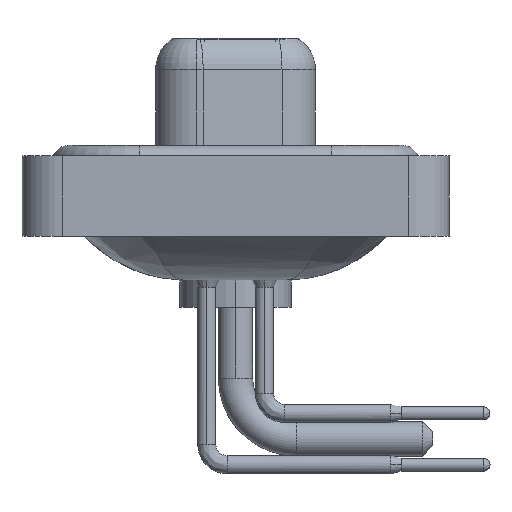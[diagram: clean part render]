
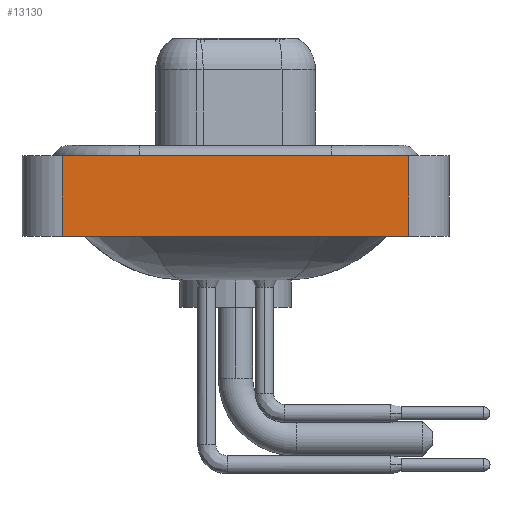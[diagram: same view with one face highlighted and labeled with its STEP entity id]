
A CAD part, left-side view. The second image highlights one B-rep face of the part: STEP entity #13130.
In plain terms, the highlighted planar face has unit normal (-1, 0, 0).
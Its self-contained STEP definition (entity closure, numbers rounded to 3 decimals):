
#79 = VECTOR ( 'NONE', #8624, 1000. ) ;
#887 = LINE ( 'NONE', #8704, #7758 ) ;
#1700 = ORIENTED_EDGE ( 'NONE', *, *, #5406, .T. ) ;
#3855 = AXIS2_PLACEMENT_3D ( 'NONE', #16000, #19322, #17631 ) ;
#4349 = EDGE_LOOP ( 'NONE', ( #1700, #16656, #8174, #11227 ) ) ;
#4826 = VECTOR ( 'NONE', #19735, 1000. ) ;
#5406 = EDGE_CURVE ( 'NONE', #7663, #13893, #16286, .T. ) ;
#5470 = CARTESIAN_POINT ( 'NONE',  ( -7.25, -8.55, 0.4 ) ) ;
#6840 = DIRECTION ( 'NONE',  ( 0., -1., 0. ) ) ;
#6926 = CARTESIAN_POINT ( 'NONE',  ( -7.25, -8.55, -3.6 ) ) ;
#7040 = CARTESIAN_POINT ( 'NONE',  ( -7.25, -8.55, 0.4 ) ) ;
#7398 = EDGE_CURVE ( 'NONE', #16177, #7663, #887, .T. ) ;
#7451 = LINE ( 'NONE', #19633, #4826 ) ;
#7663 = VERTEX_POINT ( 'NONE', #9516 ) ;
#7758 = VECTOR ( 'NONE', #13357, 1000. ) ;
#8174 = ORIENTED_EDGE ( 'NONE', *, *, #18257, .F. ) ;
#8448 = FACE_OUTER_BOUND ( 'NONE', #4349, .T. ) ;
#8624 = DIRECTION ( 'NONE',  ( 0., 0., 1. ) ) ;
#8704 = CARTESIAN_POINT ( 'NONE',  ( -7.25, -8.55, -3.6 ) ) ;
#9516 = CARTESIAN_POINT ( 'NONE',  ( -7.25, -8.55, -3.6 ) ) ;
#11227 = ORIENTED_EDGE ( 'NONE', *, *, #7398, .T. ) ;
#12423 = VERTEX_POINT ( 'NONE', #16610 ) ;
#13115 = EDGE_CURVE ( 'NONE', #12423, #13893, #14495, .T. ) ;
#13130 = ADVANCED_FACE ( 'NONE', ( #8448 ), #13192, .T. ) ;
#13192 = PLANE ( 'NONE',  #3855 ) ;
#13208 = CARTESIAN_POINT ( 'NONE',  ( -7.25, 8.55, -3.6 ) ) ;
#13357 = DIRECTION ( 'NONE',  ( 0., -1., 0. ) ) ;
#13893 = VERTEX_POINT ( 'NONE', #5470 ) ;
#14495 = LINE ( 'NONE', #7040, #14834 ) ;
#14834 = VECTOR ( 'NONE', #6840, 1000. ) ;
#16000 = CARTESIAN_POINT ( 'NONE',  ( -7.25, -8.55, -3.6 ) ) ;
#16177 = VERTEX_POINT ( 'NONE', #13208 ) ;
#16286 = LINE ( 'NONE', #6926, #79 ) ;
#16610 = CARTESIAN_POINT ( 'NONE',  ( -7.25, 8.55, 0.4 ) ) ;
#16656 = ORIENTED_EDGE ( 'NONE', *, *, #13115, .F. ) ;
#17631 = DIRECTION ( 'NONE',  ( 0., 0., 1. ) ) ;
#18257 = EDGE_CURVE ( 'NONE', #16177, #12423, #7451, .T. ) ;
#19322 = DIRECTION ( 'NONE',  ( -1., 0., 0. ) ) ;
#19633 = CARTESIAN_POINT ( 'NONE',  ( -7.25, 8.55, -3.6 ) ) ;
#19735 = DIRECTION ( 'NONE',  ( 0., 0., 1. ) ) ;
